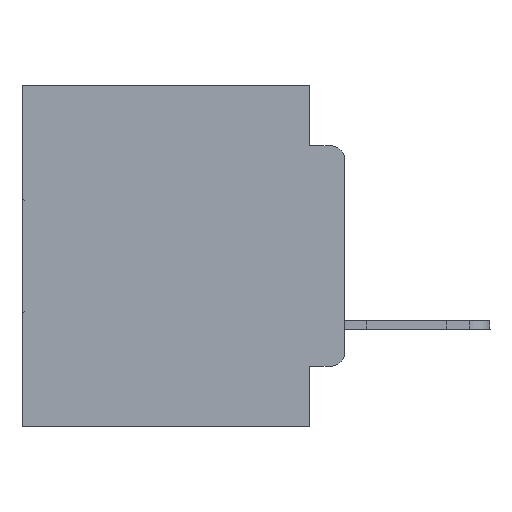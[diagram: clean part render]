
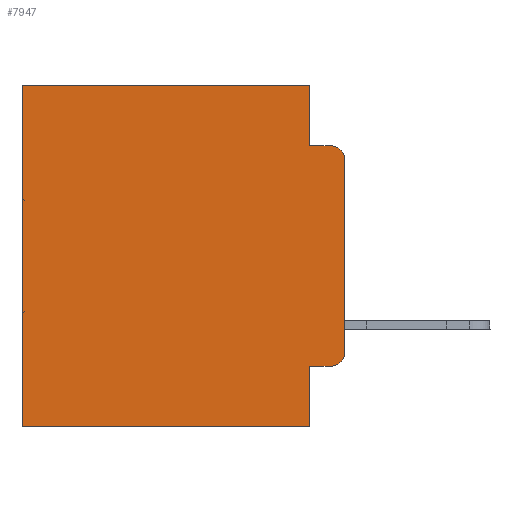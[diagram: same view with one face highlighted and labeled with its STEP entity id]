
A CAD part, left-side view. The second image highlights one B-rep face of the part: STEP entity #7947.
In plain terms, the highlighted planar face has unit normal (-1, 0, 0).
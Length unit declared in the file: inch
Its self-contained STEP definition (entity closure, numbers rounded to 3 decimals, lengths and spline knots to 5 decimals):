
#281 = VERTEX_POINT ( 'NONE', #886 ) ;
#886 = CARTESIAN_POINT ( 'NONE',  ( 0.298, 0.02, -0.4115 ) ) ;
#1194 = CARTESIAN_POINT ( 'NONE',  ( 0.298, 0.051, -0.4115 ) ) ;
#1867 = AXIS2_PLACEMENT_3D ( 'NONE', #17091, #27050, #17410 ) ;
#1974 = ORIENTED_EDGE ( 'NONE', *, *, #20029, .F. ) ;
#2063 = ORIENTED_EDGE ( 'NONE', *, *, #10556, .T. ) ;
#2131 = PLANE ( 'NONE',  #11219 ) ;
#2426 = CARTESIAN_POINT ( 'NONE',  ( 0.298, 0.473, 0. ) ) ;
#3124 = DIRECTION ( 'NONE',  ( 0., 0., -1. ) ) ;
#3565 = VECTOR ( 'NONE', #18658, 39.37008 ) ;
#4303 = CARTESIAN_POINT ( 'NONE',  ( 0.298, 0., 0. ) ) ;
#4495 = VERTEX_POINT ( 'NONE', #2426 ) ;
#4951 = ORIENTED_EDGE ( 'NONE', *, *, #19812, .F. ) ;
#6363 = ORIENTED_EDGE ( 'NONE', *, *, #19438, .T. ) ;
#6821 = CARTESIAN_POINT ( 'NONE',  ( 0.298, 0., -0.5 ) ) ;
#6992 = DIRECTION ( 'NONE',  ( 0., 0., -1. ) ) ;
#7135 = VERTEX_POINT ( 'NONE', #1194 ) ;
#7162 = LINE ( 'NONE', #14494, #31082 ) ;
#7697 = EDGE_CURVE ( 'NONE', #23445, #26341, #19427, .T. ) ;
#7947 = ADVANCED_FACE ( 'NONE', ( #24886 ), #2131, .F. ) ;
#8746 = CIRCLE ( 'NONE', #1867, 0.02 ) ;
#8797 = LINE ( 'NONE', #24084, #12555 ) ;
#9163 = CARTESIAN_POINT ( 'NONE',  ( 0.298, 0.473, 0. ) ) ;
#9543 = VERTEX_POINT ( 'NONE', #19721 ) ;
#9779 = DIRECTION ( 'NONE',  ( 1., 0., 0. ) ) ;
#9857 = VECTOR ( 'NONE', #6992, 39.37008 ) ;
#10292 = EDGE_CURVE ( 'NONE', #9543, #13134, #21122, .T. ) ;
#10556 = EDGE_CURVE ( 'NONE', #7135, #281, #17442, .T. ) ;
#10648 = CARTESIAN_POINT ( 'NONE',  ( 0.298, 0.473, -0.5 ) ) ;
#11219 = AXIS2_PLACEMENT_3D ( 'NONE', #12278, #9779, #20717 ) ;
#11285 = VECTOR ( 'NONE', #17604, 39.37008 ) ;
#12068 = CIRCLE ( 'NONE', #30621, 0.02 ) ;
#12278 = CARTESIAN_POINT ( 'NONE',  ( 0.298, 0., 0. ) ) ;
#12460 = CARTESIAN_POINT ( 'NONE',  ( 0.298, 0.051, 0. ) ) ;
#12555 = VECTOR ( 'NONE', #16139, 39.37008 ) ;
#12593 = ORIENTED_EDGE ( 'NONE', *, *, #18952, .F. ) ;
#13134 = VERTEX_POINT ( 'NONE', #10648 ) ;
#13662 = LINE ( 'NONE', #31410, #29340 ) ;
#14494 = CARTESIAN_POINT ( 'NONE',  ( 0.298, 0.051, 0. ) ) ;
#14990 = VECTOR ( 'NONE', #22258, 39.37008 ) ;
#15349 = EDGE_CURVE ( 'NONE', #20412, #4495, #13662, .T. ) ;
#15923 = CARTESIAN_POINT ( 'NONE',  ( 0.298, 0.02, -0.1085 ) ) ;
#16139 = DIRECTION ( 'NONE',  ( 0., -1., 0. ) ) ;
#16467 = VERTEX_POINT ( 'NONE', #22976 ) ;
#17091 = CARTESIAN_POINT ( 'NONE',  ( 0.298, 0.02, -0.3915 ) ) ;
#17155 = EDGE_CURVE ( 'NONE', #281, #26341, #8746, .T. ) ;
#17410 = DIRECTION ( 'NONE',  ( 0., 0., -1. ) ) ;
#17442 = LINE ( 'NONE', #27577, #11285 ) ;
#17604 = DIRECTION ( 'NONE',  ( 0., -1., 0. ) ) ;
#18259 = ORIENTED_EDGE ( 'NONE', *, *, #10292, .F. ) ;
#18658 = DIRECTION ( 'NONE',  ( 0., 0., -1. ) ) ;
#18673 = VERTEX_POINT ( 'NONE', #29447 ) ;
#18731 = EDGE_CURVE ( 'NONE', #4495, #13134, #24621, .T. ) ;
#18952 = EDGE_CURVE ( 'NONE', #18673, #16467, #8797, .T. ) ;
#19140 = CARTESIAN_POINT ( 'NONE',  ( 0.298, 0.051, 0. ) ) ;
#19245 = CARTESIAN_POINT ( 'NONE',  ( 0.298, 0., -0.1085 ) ) ;
#19427 = LINE ( 'NONE', #4303, #24848 ) ;
#19438 = EDGE_CURVE ( 'NONE', #23445, #16467, #12068, .T. ) ;
#19721 = CARTESIAN_POINT ( 'NONE',  ( 0.298, 0.051, -0.5 ) ) ;
#19812 = EDGE_CURVE ( 'NONE', #7135, #9543, #31431, .T. ) ;
#20029 = EDGE_CURVE ( 'NONE', #20412, #18673, #7162, .T. ) ;
#20412 = VERTEX_POINT ( 'NONE', #12460 ) ;
#20717 = DIRECTION ( 'NONE',  ( 0., 0., -1. ) ) ;
#21118 = DIRECTION ( 'NONE',  ( 0., 1., 0. ) ) ;
#21122 = LINE ( 'NONE', #6821, #14990 ) ;
#22144 = EDGE_LOOP ( 'NONE', ( #24993, #6363, #12593, #1974, #32460, #31002, #18259, #4951, #2063, #23732 ) ) ;
#22258 = DIRECTION ( 'NONE',  ( 0., 1., 0. ) ) ;
#22623 = DIRECTION ( 'NONE',  ( 0., 0., -1. ) ) ;
#22976 = CARTESIAN_POINT ( 'NONE',  ( 0.298, 0.02, -0.0885 ) ) ;
#23445 = VERTEX_POINT ( 'NONE', #19245 ) ;
#23732 = ORIENTED_EDGE ( 'NONE', *, *, #17155, .T. ) ;
#24084 = CARTESIAN_POINT ( 'NONE',  ( 0.298, 0.051, -0.0885 ) ) ;
#24621 = LINE ( 'NONE', #9163, #9857 ) ;
#24848 = VECTOR ( 'NONE', #29403, 39.37008 ) ;
#24886 = FACE_OUTER_BOUND ( 'NONE', #22144, .T. ) ;
#24993 = ORIENTED_EDGE ( 'NONE', *, *, #7697, .F. ) ;
#26341 = VERTEX_POINT ( 'NONE', #30730 ) ;
#27050 = DIRECTION ( 'NONE',  ( -1., 0., 0. ) ) ;
#27577 = CARTESIAN_POINT ( 'NONE',  ( 0.298, 0.051, -0.4115 ) ) ;
#29340 = VECTOR ( 'NONE', #21118, 39.37008 ) ;
#29403 = DIRECTION ( 'NONE',  ( 0., 0., -1. ) ) ;
#29447 = CARTESIAN_POINT ( 'NONE',  ( 0.298, 0.051, -0.0885 ) ) ;
#30621 = AXIS2_PLACEMENT_3D ( 'NONE', #15923, #30858, #3124 ) ;
#30730 = CARTESIAN_POINT ( 'NONE',  ( 0.298, 0., -0.3915 ) ) ;
#30858 = DIRECTION ( 'NONE',  ( -1., 0., 0. ) ) ;
#31002 = ORIENTED_EDGE ( 'NONE', *, *, #18731, .T. ) ;
#31082 = VECTOR ( 'NONE', #22623, 39.37008 ) ;
#31410 = CARTESIAN_POINT ( 'NONE',  ( 0.298, 0., 0. ) ) ;
#31431 = LINE ( 'NONE', #19140, #3565 ) ;
#32460 = ORIENTED_EDGE ( 'NONE', *, *, #15349, .T. ) ;
